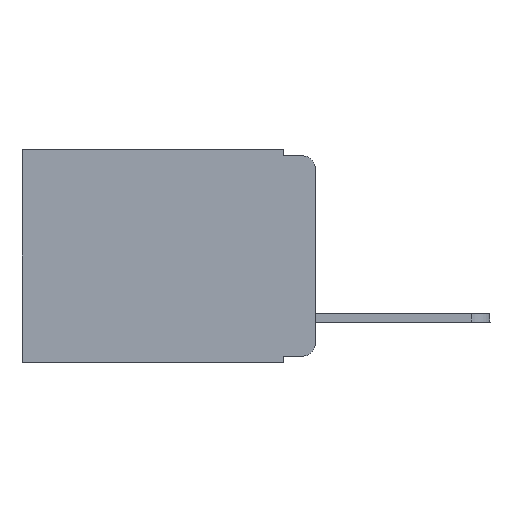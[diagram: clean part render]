
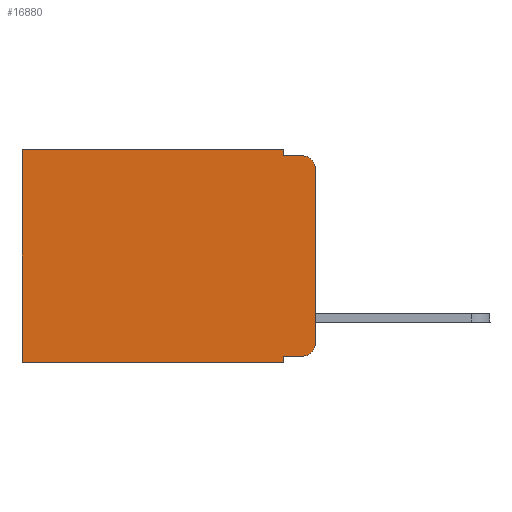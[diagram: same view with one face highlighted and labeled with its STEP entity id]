
A CAD part, left-side view. The second image highlights one B-rep face of the part: STEP entity #16880.
In plain terms, the highlighted planar face has unit normal (-1, 0, 0).
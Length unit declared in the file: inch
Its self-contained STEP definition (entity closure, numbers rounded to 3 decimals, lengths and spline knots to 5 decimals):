
#224 = EDGE_CURVE ( 'NONE', #7702, #13183, #8102, .T. ) ;
#254 = DIRECTION ( 'NONE',  ( 1., 0., 0. ) ) ;
#294 = ORIENTED_EDGE ( 'NONE', *, *, #224, .F. ) ;
#318 = EDGE_CURVE ( 'NONE', #1718, #8131, #11788, .T. ) ;
#401 = VERTEX_POINT ( 'NONE', #14634 ) ;
#461 = ORIENTED_EDGE ( 'NONE', *, *, #4793, .F. ) ;
#470 = AXIS2_PLACEMENT_3D ( 'NONE', #8393, #254, #12521 ) ;
#491 = DIRECTION ( 'NONE',  ( -1., 0., 0. ) ) ;
#606 = ORIENTED_EDGE ( 'NONE', *, *, #6290, .T. ) ;
#616 = LINE ( 'NONE', #9711, #11307 ) ;
#1470 = CARTESIAN_POINT ( 'NONE',  ( 0.298, 0.02, -0.333 ) ) ;
#1558 = CARTESIAN_POINT ( 'NONE',  ( 0.298, 0., -0.313 ) ) ;
#1718 = VERTEX_POINT ( 'NONE', #11991 ) ;
#2020 = EDGE_CURVE ( 'NONE', #7129, #14161, #3914, .T. ) ;
#2203 = ORIENTED_EDGE ( 'NONE', *, *, #318, .F. ) ;
#2623 = DIRECTION ( 'NONE',  ( 0., 0., -1. ) ) ;
#2958 = VERTEX_POINT ( 'NONE', #17142 ) ;
#3327 = CARTESIAN_POINT ( 'NONE',  ( 0.298, 0.02, -0.313 ) ) ;
#3379 = EDGE_CURVE ( 'NONE', #401, #1718, #11517, .T. ) ;
#3554 = EDGE_CURVE ( 'NONE', #7702, #14022, #616, .T. ) ;
#3645 = AXIS2_PLACEMENT_3D ( 'NONE', #3327, #491, #14459 ) ;
#3823 = CARTESIAN_POINT ( 'NONE',  ( 0.298, 0.051, 0. ) ) ;
#3914 = CIRCLE ( 'NONE', #3645, 0.02 ) ;
#4119 = LINE ( 'NONE', #16863, #8520 ) ;
#4537 = VECTOR ( 'NONE', #13313, 39.37008 ) ;
#4606 = DIRECTION ( 'NONE',  ( 0., 0., -1. ) ) ;
#4672 = CARTESIAN_POINT ( 'NONE',  ( 0.298, 0., -0.343 ) ) ;
#4793 = EDGE_CURVE ( 'NONE', #13183, #2958, #17386, .T. ) ;
#5093 = LINE ( 'NONE', #12429, #15393 ) ;
#5337 = ORIENTED_EDGE ( 'NONE', *, *, #10533, .T. ) ;
#6110 = VECTOR ( 'NONE', #4606, 39.37008 ) ;
#6290 = EDGE_CURVE ( 'NONE', #14022, #8131, #5093, .T. ) ;
#6766 = DIRECTION ( 'NONE',  ( 0., 0., -1. ) ) ;
#7129 = VERTEX_POINT ( 'NONE', #1470 ) ;
#7702 = VERTEX_POINT ( 'NONE', #15384 ) ;
#7855 = ORIENTED_EDGE ( 'NONE', *, *, #10769, .T. ) ;
#8102 = LINE ( 'NONE', #11404, #6110 ) ;
#8131 = VERTEX_POINT ( 'NONE', #12075 ) ;
#8309 = CARTESIAN_POINT ( 'NONE',  ( 0.298, 0.051, -0.01 ) ) ;
#8368 = DIRECTION ( 'NONE',  ( 0., 1., 0. ) ) ;
#8393 = CARTESIAN_POINT ( 'NONE',  ( 0.298, 0., 0. ) ) ;
#8520 = VECTOR ( 'NONE', #12782, 39.37008 ) ;
#8809 = AXIS2_PLACEMENT_3D ( 'NONE', #9262, #9206, #14743 ) ;
#9206 = DIRECTION ( 'NONE',  ( -1., 0., 0. ) ) ;
#9262 = CARTESIAN_POINT ( 'NONE',  ( 0.298, 0.02, -0.03 ) ) ;
#9534 = VECTOR ( 'NONE', #13920, 39.37008 ) ;
#9565 = VERTEX_POINT ( 'NONE', #11750 ) ;
#9711 = CARTESIAN_POINT ( 'NONE',  ( 0.298, 0., 0. ) ) ;
#10533 = EDGE_CURVE ( 'NONE', #9565, #2958, #16420, .T. ) ;
#10769 = EDGE_CURVE ( 'NONE', #401, #7129, #17076, .T. ) ;
#10822 = CARTESIAN_POINT ( 'NONE',  ( 0.298, 0.051, -0.01 ) ) ;
#11307 = VECTOR ( 'NONE', #8368, 39.37008 ) ;
#11404 = CARTESIAN_POINT ( 'NONE',  ( 0.298, 0.051, 0. ) ) ;
#11517 = LINE ( 'NONE', #3823, #16546 ) ;
#11613 = VECTOR ( 'NONE', #12082, 39.37008 ) ;
#11750 = CARTESIAN_POINT ( 'NONE',  ( 0.298, 0., -0.03 ) ) ;
#11788 = LINE ( 'NONE', #4672, #4537 ) ;
#11991 = CARTESIAN_POINT ( 'NONE',  ( 0.298, 0.051, -0.343 ) ) ;
#12075 = CARTESIAN_POINT ( 'NONE',  ( 0.298, 0.473, -0.343 ) ) ;
#12082 = DIRECTION ( 'NONE',  ( 0., -1., 0. ) ) ;
#12429 = CARTESIAN_POINT ( 'NONE',  ( 0.298, 0.473, 0. ) ) ;
#12464 = EDGE_CURVE ( 'NONE', #9565, #14161, #4119, .T. ) ;
#12521 = DIRECTION ( 'NONE',  ( 0., 0., -1. ) ) ;
#12700 = PLANE ( 'NONE',  #470 ) ;
#12782 = DIRECTION ( 'NONE',  ( 0., 0., -1. ) ) ;
#12814 = FACE_OUTER_BOUND ( 'NONE', #16529, .T. ) ;
#13183 = VERTEX_POINT ( 'NONE', #10822 ) ;
#13313 = DIRECTION ( 'NONE',  ( 0., 1., 0. ) ) ;
#13920 = DIRECTION ( 'NONE',  ( 0., -1., 0. ) ) ;
#14022 = VERTEX_POINT ( 'NONE', #17521 ) ;
#14111 = ORIENTED_EDGE ( 'NONE', *, *, #3379, .F. ) ;
#14161 = VERTEX_POINT ( 'NONE', #1558 ) ;
#14459 = DIRECTION ( 'NONE',  ( 0., 0., -1. ) ) ;
#14634 = CARTESIAN_POINT ( 'NONE',  ( 0.298, 0.051, -0.333 ) ) ;
#14743 = DIRECTION ( 'NONE',  ( 0., 0., -1. ) ) ;
#15384 = CARTESIAN_POINT ( 'NONE',  ( 0.298, 0.051, 0. ) ) ;
#15393 = VECTOR ( 'NONE', #6766, 39.37008 ) ;
#16278 = CARTESIAN_POINT ( 'NONE',  ( 0.298, 0.051, -0.333 ) ) ;
#16420 = CIRCLE ( 'NONE', #8809, 0.02 ) ;
#16529 = EDGE_LOOP ( 'NONE', ( #17825, #5337, #461, #294, #17672, #606, #2203, #14111, #7855, #17085 ) ) ;
#16546 = VECTOR ( 'NONE', #2623, 39.37008 ) ;
#16863 = CARTESIAN_POINT ( 'NONE',  ( 0.298, 0., 0. ) ) ;
#16880 = ADVANCED_FACE ( 'NONE', ( #12814 ), #12700, .F. ) ;
#17076 = LINE ( 'NONE', #16278, #11613 ) ;
#17085 = ORIENTED_EDGE ( 'NONE', *, *, #2020, .T. ) ;
#17142 = CARTESIAN_POINT ( 'NONE',  ( 0.298, 0.02, -0.01 ) ) ;
#17386 = LINE ( 'NONE', #8309, #9534 ) ;
#17521 = CARTESIAN_POINT ( 'NONE',  ( 0.298, 0.473, 0. ) ) ;
#17672 = ORIENTED_EDGE ( 'NONE', *, *, #3554, .T. ) ;
#17825 = ORIENTED_EDGE ( 'NONE', *, *, #12464, .F. ) ;
